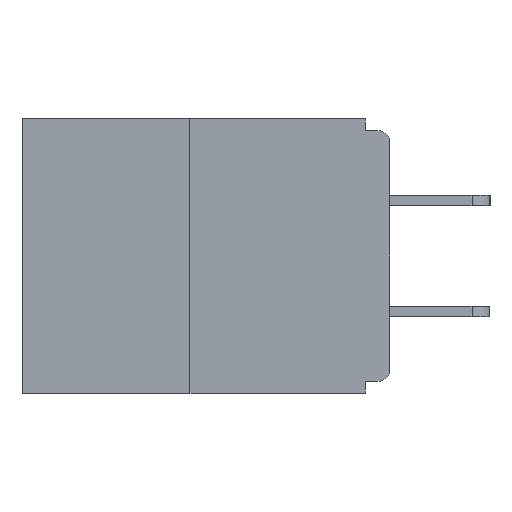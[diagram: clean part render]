
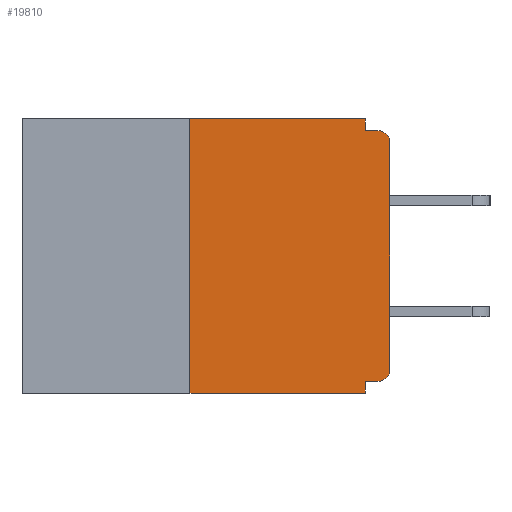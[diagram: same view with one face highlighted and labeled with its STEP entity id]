
A CAD part, left-side view. The second image highlights one B-rep face of the part: STEP entity #19810.
In plain terms, the highlighted planar face has unit normal (-1, 0, 0).
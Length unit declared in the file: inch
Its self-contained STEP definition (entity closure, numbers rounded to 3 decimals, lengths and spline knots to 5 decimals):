
#195 = FACE_OUTER_BOUND ( 'NONE', #8215, .T. ) ;
#1561 = VERTEX_POINT ( 'NONE', #19477 ) ;
#2887 = ORIENTED_EDGE ( 'NONE', *, *, #11469, .F. ) ;
#2988 = LINE ( 'NONE', #12007, #17777 ) ;
#3112 = VERTEX_POINT ( 'NONE', #11260 ) ;
#3390 = ORIENTED_EDGE ( 'NONE', *, *, #4615, .T. ) ;
#4061 = VERTEX_POINT ( 'NONE', #13480 ) ;
#4075 = LINE ( 'NONE', #22037, #13481 ) ;
#4079 = AXIS2_PLACEMENT_3D ( 'NONE', #14770, #16502, #7926 ) ;
#4548 = DIRECTION ( 'NONE',  ( 0., 0., -1. ) ) ;
#4615 = EDGE_CURVE ( 'NONE', #3112, #1561, #8243, .T. ) ;
#4630 = ORIENTED_EDGE ( 'NONE', *, *, #11971, .F. ) ;
#4736 = VERTEX_POINT ( 'NONE', #7754 ) ;
#4901 = DIRECTION ( 'NONE',  ( 0., 0., 1. ) ) ;
#5041 = DIRECTION ( 'NONE',  ( 0., 0., -1. ) ) ;
#5342 = ORIENTED_EDGE ( 'NONE', *, *, #21705, .F. ) ;
#5754 = EDGE_CURVE ( 'NONE', #16276, #4736, #14618, .T. ) ;
#5776 = EDGE_CURVE ( 'NONE', #3112, #4061, #19189, .T. ) ;
#6147 = DIRECTION ( 'NONE',  ( -1., 0., 0. ) ) ;
#6649 = DIRECTION ( 'NONE',  ( 0., -1., 0. ) ) ;
#6694 = VERTEX_POINT ( 'NONE', #21215 ) ;
#7754 = CARTESIAN_POINT ( 'NONE',  ( 0., 0., -0.313 ) ) ;
#7926 = DIRECTION ( 'NONE',  ( 0., 0., -1. ) ) ;
#7966 = EDGE_CURVE ( 'NONE', #4061, #17323, #2988, .T. ) ;
#8046 = ORIENTED_EDGE ( 'NONE', *, *, #5754, .T. ) ;
#8215 = EDGE_LOOP ( 'NONE', ( #11136, #17691, #3390, #5342, #2887, #8046, #19321, #12246, #4630, #15603 ) ) ;
#8243 = LINE ( 'NONE', #18508, #21409 ) ;
#8360 = VERTEX_POINT ( 'NONE', #19867 ) ;
#8657 = LINE ( 'NONE', #10487, #14278 ) ;
#9248 = VECTOR ( 'NONE', #4901, 39.37008 ) ;
#9360 = LINE ( 'NONE', #20611, #14205 ) ;
#10308 = VERTEX_POINT ( 'NONE', #21587 ) ;
#10408 = CIRCLE ( 'NONE', #11262, 0.015 ) ;
#10487 = CARTESIAN_POINT ( 'NONE',  ( 0., 0., 0. ) ) ;
#11136 = ORIENTED_EDGE ( 'NONE', *, *, #7966, .F. ) ;
#11214 = DIRECTION ( 'NONE',  ( 0., 1., 0. ) ) ;
#11260 = CARTESIAN_POINT ( 'NONE',  ( 0., 0.25, -0.343 ) ) ;
#11262 = AXIS2_PLACEMENT_3D ( 'NONE', #14716, #6147, #4548 ) ;
#11469 = EDGE_CURVE ( 'NONE', #16276, #6694, #18877, .T. ) ;
#11899 = VECTOR ( 'NONE', #11214, 39.37008 ) ;
#11971 = EDGE_CURVE ( 'NONE', #8360, #20207, #4075, .T. ) ;
#12007 = CARTESIAN_POINT ( 'NONE',  ( 0., 0.46, 0. ) ) ;
#12060 = DIRECTION ( 'NONE',  ( 0., 0., -1. ) ) ;
#12246 = ORIENTED_EDGE ( 'NONE', *, *, #21201, .T. ) ;
#12301 = CARTESIAN_POINT ( 'NONE',  ( 0., 0.031, -0.343 ) ) ;
#13152 = DIRECTION ( 'NONE',  ( 0., 0., -1. ) ) ;
#13310 = CARTESIAN_POINT ( 'NONE',  ( 0., 0.015, -0.313 ) ) ;
#13463 = DIRECTION ( 'NONE',  ( -1., 0., 0. ) ) ;
#13480 = CARTESIAN_POINT ( 'NONE',  ( 0., 0.25, 0. ) ) ;
#13481 = VECTOR ( 'NONE', #6649, 39.37008 ) ;
#14205 = VECTOR ( 'NONE', #5041, 39.37008 ) ;
#14278 = VECTOR ( 'NONE', #15808, 39.37008 ) ;
#14585 = AXIS2_PLACEMENT_3D ( 'NONE', #13310, #13463, #13152 ) ;
#14618 = CIRCLE ( 'NONE', #14585, 0.015 ) ;
#14716 = CARTESIAN_POINT ( 'NONE',  ( 0., 0.015, -0.03 ) ) ;
#14770 = CARTESIAN_POINT ( 'NONE',  ( 0., 0.46, 0. ) ) ;
#15603 = ORIENTED_EDGE ( 'NONE', *, *, #20189, .F. ) ;
#15808 = DIRECTION ( 'NONE',  ( 0., 0., 1. ) ) ;
#16276 = VERTEX_POINT ( 'NONE', #16668 ) ;
#16502 = DIRECTION ( 'NONE',  ( 1., 0., 0. ) ) ;
#16668 = CARTESIAN_POINT ( 'NONE',  ( 0., 0.015, -0.328 ) ) ;
#16910 = CARTESIAN_POINT ( 'NONE',  ( 0., 0.015, -0.015 ) ) ;
#17110 = DIRECTION ( 'NONE',  ( 0., -1., 0. ) ) ;
#17323 = VERTEX_POINT ( 'NONE', #21810 ) ;
#17691 = ORIENTED_EDGE ( 'NONE', *, *, #5776, .F. ) ;
#17777 = VECTOR ( 'NONE', #17110, 39.37008 ) ;
#18194 = EDGE_CURVE ( 'NONE', #4736, #10308, #8657, .T. ) ;
#18491 = CARTESIAN_POINT ( 'NONE',  ( 0., 0.25, 0. ) ) ;
#18508 = CARTESIAN_POINT ( 'NONE',  ( 0., 0.46, -0.343 ) ) ;
#18877 = LINE ( 'NONE', #21548, #11899 ) ;
#19189 = LINE ( 'NONE', #18491, #9248 ) ;
#19321 = ORIENTED_EDGE ( 'NONE', *, *, #18194, .T. ) ;
#19477 = CARTESIAN_POINT ( 'NONE',  ( 0., 0.031, -0.343 ) ) ;
#19493 = VECTOR ( 'NONE', #12060, 39.37008 ) ;
#19810 = ADVANCED_FACE ( 'NONE', ( #195 ), #20027, .F. ) ;
#19867 = CARTESIAN_POINT ( 'NONE',  ( 0., 0.031, -0.015 ) ) ;
#20027 = PLANE ( 'NONE',  #4079 ) ;
#20098 = DIRECTION ( 'NONE',  ( 0., -1., 0. ) ) ;
#20189 = EDGE_CURVE ( 'NONE', #17323, #8360, #9360, .T. ) ;
#20207 = VERTEX_POINT ( 'NONE', #16910 ) ;
#20598 = LINE ( 'NONE', #12301, #19493 ) ;
#20611 = CARTESIAN_POINT ( 'NONE',  ( 0., 0.031, 0. ) ) ;
#21201 = EDGE_CURVE ( 'NONE', #10308, #20207, #10408, .T. ) ;
#21215 = CARTESIAN_POINT ( 'NONE',  ( 0., 0.031, -0.328 ) ) ;
#21409 = VECTOR ( 'NONE', #20098, 39.37008 ) ;
#21548 = CARTESIAN_POINT ( 'NONE',  ( 0., 0., -0.328 ) ) ;
#21587 = CARTESIAN_POINT ( 'NONE',  ( 0., 0., -0.03 ) ) ;
#21705 = EDGE_CURVE ( 'NONE', #6694, #1561, #20598, .T. ) ;
#21810 = CARTESIAN_POINT ( 'NONE',  ( 0., 0.031, 0. ) ) ;
#22037 = CARTESIAN_POINT ( 'NONE',  ( 0., 0., -0.015 ) ) ;
